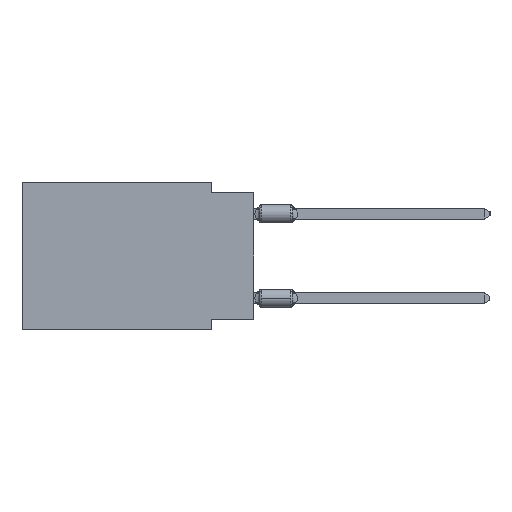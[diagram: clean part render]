
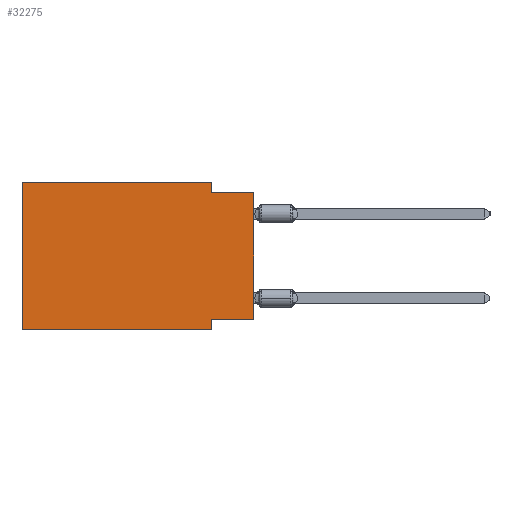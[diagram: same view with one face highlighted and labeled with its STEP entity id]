
A CAD part, left-side view. The second image highlights one B-rep face of the part: STEP entity #32275.
In plain terms, the highlighted planar face has unit normal (-1, 0, 0).
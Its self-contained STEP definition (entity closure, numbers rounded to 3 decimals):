
#744 = DIRECTION ( 'NONE',  ( 0., 0., -1. ) ) ;
#1907 = EDGE_LOOP ( 'NONE', ( #23533, #20766, #5404, #3333, #34706, #7908, #44422, #6927 ) ) ;
#2290 = VECTOR ( 'NONE', #20095, 1000. ) ;
#2568 = LINE ( 'NONE', #19945, #30948 ) ;
#3333 = ORIENTED_EDGE ( 'NONE', *, *, #42581, .F. ) ;
#4398 = LINE ( 'NONE', #29527, #31075 ) ;
#4531 = CARTESIAN_POINT ( 'NONE',  ( 0., 2.54, -8.89 ) ) ;
#5065 = PLANE ( 'NONE',  #27777 ) ;
#5296 = FACE_OUTER_BOUND ( 'NONE', #1907, .T. ) ;
#5404 = ORIENTED_EDGE ( 'NONE', *, *, #14569, .F. ) ;
#5858 = CARTESIAN_POINT ( 'NONE',  ( 0., 2.54, -8.89 ) ) ;
#6424 = VERTEX_POINT ( 'NONE', #8231 ) ;
#6927 = ORIENTED_EDGE ( 'NONE', *, *, #31426, .F. ) ;
#7636 = EDGE_CURVE ( 'NONE', #16661, #33739, #23309, .T. ) ;
#7908 = ORIENTED_EDGE ( 'NONE', *, *, #7636, .T. ) ;
#8231 = CARTESIAN_POINT ( 'NONE',  ( 0., 2.54, -0.635 ) ) ;
#8896 = CARTESIAN_POINT ( 'NONE',  ( 0., 0., -8.255 ) ) ;
#12598 = CARTESIAN_POINT ( 'NONE',  ( 0., 13.97, 0. ) ) ;
#12715 = LINE ( 'NONE', #40122, #20792 ) ;
#12724 = LINE ( 'NONE', #5858, #22944 ) ;
#13026 = DIRECTION ( 'NONE',  ( 0., -1., 0. ) ) ;
#14569 = EDGE_CURVE ( 'NONE', #43618, #6424, #4398, .T. ) ;
#15807 = LINE ( 'NONE', #29728, #29853 ) ;
#16661 = VERTEX_POINT ( 'NONE', #35967 ) ;
#17314 = EDGE_CURVE ( 'NONE', #6424, #30534, #26523, .T. ) ;
#17765 = EDGE_CURVE ( 'NONE', #26043, #30534, #12715, .T. ) ;
#19026 = DIRECTION ( 'NONE',  ( 1., 0., 0. ) ) ;
#19459 = CARTESIAN_POINT ( 'NONE',  ( 0., 0., -0.635 ) ) ;
#19816 = DIRECTION ( 'NONE',  ( 0., 0., -1. ) ) ;
#19945 = CARTESIAN_POINT ( 'NONE',  ( 0., 13.97, 0. ) ) ;
#20095 = DIRECTION ( 'NONE',  ( 0., 1., 0. ) ) ;
#20766 = ORIENTED_EDGE ( 'NONE', *, *, #17314, .F. ) ;
#20792 = VECTOR ( 'NONE', #41026, 1000. ) ;
#22944 = VECTOR ( 'NONE', #19816, 1000. ) ;
#22963 = CARTESIAN_POINT ( 'NONE',  ( 0., 0., -0.635 ) ) ;
#23309 = LINE ( 'NONE', #37001, #25972 ) ;
#23533 = ORIENTED_EDGE ( 'NONE', *, *, #17765, .T. ) ;
#24047 = EDGE_CURVE ( 'NONE', #16661, #33481, #15807, .T. ) ;
#25845 = DIRECTION ( 'NONE',  ( 0., -1., 0. ) ) ;
#25972 = VECTOR ( 'NONE', #13026, 1000. ) ;
#26043 = VERTEX_POINT ( 'NONE', #38848 ) ;
#26523 = LINE ( 'NONE', #19459, #27654 ) ;
#27654 = VECTOR ( 'NONE', #25845, 1000. ) ;
#27777 = AXIS2_PLACEMENT_3D ( 'NONE', #33164, #19026, #43688 ) ;
#29527 = CARTESIAN_POINT ( 'NONE',  ( 0., 2.54, 0. ) ) ;
#29728 = CARTESIAN_POINT ( 'NONE',  ( 0., 13.97, 0. ) ) ;
#29853 = VECTOR ( 'NONE', #41139, 1000. ) ;
#30534 = VERTEX_POINT ( 'NONE', #22963 ) ;
#30744 = VERTEX_POINT ( 'NONE', #38874 ) ;
#30948 = VECTOR ( 'NONE', #40948, 1000. ) ;
#31075 = VECTOR ( 'NONE', #744, 1000. ) ;
#31426 = EDGE_CURVE ( 'NONE', #26043, #30744, #34220, .T. ) ;
#32275 = ADVANCED_FACE ( 'NONE', ( #5296 ), #5065, .F. ) ;
#33164 = CARTESIAN_POINT ( 'NONE',  ( 0., 13.97, 0. ) ) ;
#33481 = VERTEX_POINT ( 'NONE', #12598 ) ;
#33739 = VERTEX_POINT ( 'NONE', #4531 ) ;
#33971 = CARTESIAN_POINT ( 'NONE',  ( 0., 2.54, 0. ) ) ;
#34220 = LINE ( 'NONE', #8896, #2290 ) ;
#34706 = ORIENTED_EDGE ( 'NONE', *, *, #24047, .F. ) ;
#35700 = EDGE_CURVE ( 'NONE', #30744, #33739, #12724, .T. ) ;
#35967 = CARTESIAN_POINT ( 'NONE',  ( 0., 13.97, -8.89 ) ) ;
#37001 = CARTESIAN_POINT ( 'NONE',  ( 0., 13.97, -8.89 ) ) ;
#38848 = CARTESIAN_POINT ( 'NONE',  ( 0., 0., -8.255 ) ) ;
#38874 = CARTESIAN_POINT ( 'NONE',  ( 0., 2.54, -8.255 ) ) ;
#40122 = CARTESIAN_POINT ( 'NONE',  ( 0., 0., 0. ) ) ;
#40948 = DIRECTION ( 'NONE',  ( 0., -1., 0. ) ) ;
#41026 = DIRECTION ( 'NONE',  ( 0., 0., 1. ) ) ;
#41139 = DIRECTION ( 'NONE',  ( 0., 0., 1. ) ) ;
#42581 = EDGE_CURVE ( 'NONE', #33481, #43618, #2568, .T. ) ;
#43618 = VERTEX_POINT ( 'NONE', #33971 ) ;
#43688 = DIRECTION ( 'NONE',  ( 0., 0., -1. ) ) ;
#44422 = ORIENTED_EDGE ( 'NONE', *, *, #35700, .F. ) ;
